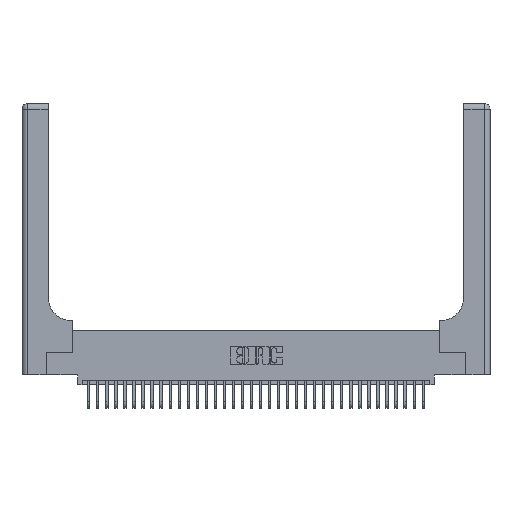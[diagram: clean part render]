
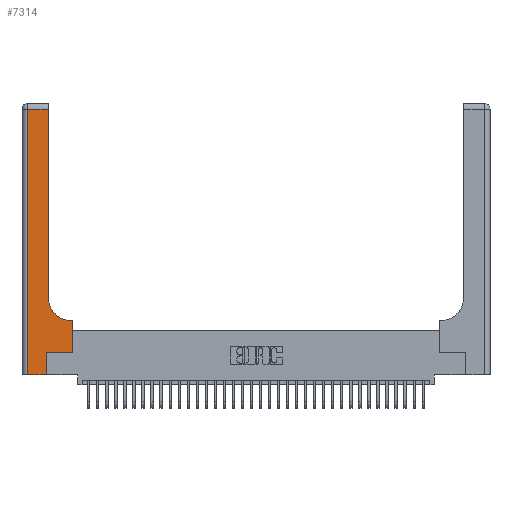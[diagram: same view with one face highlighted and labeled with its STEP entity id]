
A CAD part, top view. The second image highlights one B-rep face of the part: STEP entity #7314.
In plain terms, the highlighted planar face has unit normal (0, 0, 1).
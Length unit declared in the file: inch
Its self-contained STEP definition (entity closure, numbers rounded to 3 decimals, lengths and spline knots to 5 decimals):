
#1016 = ORIENTED_EDGE ( 'NONE', *, *, #7692, .T. ) ;
#1491 = CARTESIAN_POINT ( 'NONE',  ( 0.269, 0.25, 0.37 ) ) ;
#2041 = VERTEX_POINT ( 'NONE', #24677 ) ;
#3075 = EDGE_CURVE ( 'NONE', #2041, #9652, #34092, .T. ) ;
#4095 = DIRECTION ( 'NONE',  ( 1., 0., 0. ) ) ;
#4348 = LINE ( 'NONE', #24322, #18525 ) ;
#5325 = CARTESIAN_POINT ( 'NONE',  ( 0.5415, 0.85, 0.37 ) ) ;
#5831 = ORIENTED_EDGE ( 'NONE', *, *, #3075, .T. ) ;
#7272 = CARTESIAN_POINT ( 'NONE',  ( 0.5585, 0.25, 0.37 ) ) ;
#7314 = ADVANCED_FACE ( 'NONE', ( #29345 ), #9609, .F. ) ;
#7692 = EDGE_CURVE ( 'NONE', #11512, #23605, #4348, .T. ) ;
#8021 = DIRECTION ( 'NONE',  ( 1., 0., 0. ) ) ;
#8055 = ORIENTED_EDGE ( 'NONE', *, *, #15020, .T. ) ;
#8396 = DIRECTION ( 'NONE',  ( -1., 0., 0. ) ) ;
#9609 = PLANE ( 'NONE',  #15354 ) ;
#9652 = VERTEX_POINT ( 'NONE', #24457 ) ;
#10002 = VECTOR ( 'NONE', #10440, 39.37008 ) ;
#10163 = VECTOR ( 'NONE', #30963, 39.37008 ) ;
#10440 = DIRECTION ( 'NONE',  ( -1., 0., 0. ) ) ;
#11512 = VERTEX_POINT ( 'NONE', #14588 ) ;
#12380 = ORIENTED_EDGE ( 'NONE', *, *, #18925, .T. ) ;
#12418 = EDGE_CURVE ( 'NONE', #18332, #13739, #17398, .T. ) ;
#12611 = CARTESIAN_POINT ( 'NONE',  ( 0.269, 0., 0.37 ) ) ;
#12645 = DIRECTION ( 'NONE',  ( 0., 1., 0. ) ) ;
#13209 = CARTESIAN_POINT ( 'NONE',  ( 0., 2.94, 0.37 ) ) ;
#13588 = ORIENTED_EDGE ( 'NONE', *, *, #29686, .T. ) ;
#13739 = VERTEX_POINT ( 'NONE', #17241 ) ;
#14588 = CARTESIAN_POINT ( 'NONE',  ( 0.5585, 0.6, 0.37 ) ) ;
#14940 = CARTESIAN_POINT ( 'NONE',  ( 0., 3., 0.37 ) ) ;
#15020 = EDGE_CURVE ( 'NONE', #29560, #11512, #29086, .T. ) ;
#15139 = CARTESIAN_POINT ( 'NONE',  ( 0.06, 2.94, 0.37 ) ) ;
#15354 = AXIS2_PLACEMENT_3D ( 'NONE', #14940, #33501, #17611 ) ;
#15803 = DIRECTION ( 'NONE',  ( 0., 1., 0. ) ) ;
#16868 = CIRCLE ( 'NONE', #20278, 0.25 ) ;
#17241 = CARTESIAN_POINT ( 'NONE',  ( 0.269, 0.25, 0.37 ) ) ;
#17398 = LINE ( 'NONE', #26371, #30698 ) ;
#17611 = DIRECTION ( 'NONE',  ( -1., 0., 0. ) ) ;
#17655 = VECTOR ( 'NONE', #27578, 39.37008 ) ;
#17733 = CARTESIAN_POINT ( 'NONE',  ( 0.06, 3., 0.37 ) ) ;
#18332 = VERTEX_POINT ( 'NONE', #12611 ) ;
#18525 = VECTOR ( 'NONE', #8396, 39.37008 ) ;
#18925 = EDGE_CURVE ( 'NONE', #24624, #18332, #33434, .T. ) ;
#20275 = CARTESIAN_POINT ( 'NONE',  ( 0.2915, 3., 0.37 ) ) ;
#20278 = AXIS2_PLACEMENT_3D ( 'NONE', #5325, #23956, #8021 ) ;
#20395 = ORIENTED_EDGE ( 'NONE', *, *, #12418, .T. ) ;
#22029 = VECTOR ( 'NONE', #12645, 39.37008 ) ;
#23605 = VERTEX_POINT ( 'NONE', #27385 ) ;
#23956 = DIRECTION ( 'NONE',  ( 0., 0., -1. ) ) ;
#24119 = EDGE_CURVE ( 'NONE', #9652, #32865, #24959, .T. ) ;
#24322 = CARTESIAN_POINT ( 'NONE',  ( 0.2915, 0.6, 0.37 ) ) ;
#24457 = CARTESIAN_POINT ( 'NONE',  ( 0.2915, 2.94, 0.37 ) ) ;
#24624 = VERTEX_POINT ( 'NONE', #28833 ) ;
#24677 = CARTESIAN_POINT ( 'NONE',  ( 0.2915, 0.85, 0.37 ) ) ;
#24959 = LINE ( 'NONE', #13209, #10002 ) ;
#26371 = CARTESIAN_POINT ( 'NONE',  ( 0.269, 0., 0.37 ) ) ;
#26693 = EDGE_LOOP ( 'NONE', ( #5831, #28457, #27850, #12380, #20395, #13588, #8055, #1016, #27138 ) ) ;
#27138 = ORIENTED_EDGE ( 'NONE', *, *, #30465, .T. ) ;
#27385 = CARTESIAN_POINT ( 'NONE',  ( 0.5415, 0.6, 0.37 ) ) ;
#27474 = CARTESIAN_POINT ( 'NONE',  ( 0.5585, 0.25, 0.37 ) ) ;
#27578 = DIRECTION ( 'NONE',  ( 1., 0., 0. ) ) ;
#27850 = ORIENTED_EDGE ( 'NONE', *, *, #31530, .T. ) ;
#28457 = ORIENTED_EDGE ( 'NONE', *, *, #24119, .T. ) ;
#28558 = VECTOR ( 'NONE', #4095, 39.37008 ) ;
#28833 = CARTESIAN_POINT ( 'NONE',  ( 0.06, 0., 0.37 ) ) ;
#29086 = LINE ( 'NONE', #7272, #22029 ) ;
#29345 = FACE_OUTER_BOUND ( 'NONE', #26693, .T. ) ;
#29394 = LINE ( 'NONE', #1491, #28558 ) ;
#29560 = VERTEX_POINT ( 'NONE', #27474 ) ;
#29686 = EDGE_CURVE ( 'NONE', #13739, #29560, #29394, .T. ) ;
#30465 = EDGE_CURVE ( 'NONE', #23605, #2041, #16868, .T. ) ;
#30488 = LINE ( 'NONE', #17733, #10163 ) ;
#30698 = VECTOR ( 'NONE', #15803, 39.37008 ) ;
#30963 = DIRECTION ( 'NONE',  ( 0., -1., 0. ) ) ;
#31530 = EDGE_CURVE ( 'NONE', #32865, #24624, #30488, .T. ) ;
#32865 = VERTEX_POINT ( 'NONE', #15139 ) ;
#32911 = CARTESIAN_POINT ( 'NONE',  ( 0., 0., 0.37 ) ) ;
#33266 = VECTOR ( 'NONE', #33508, 39.37008 ) ;
#33434 = LINE ( 'NONE', #32911, #17655 ) ;
#33501 = DIRECTION ( 'NONE',  ( 0., 0., -1. ) ) ;
#33508 = DIRECTION ( 'NONE',  ( 0., 1., 0. ) ) ;
#34092 = LINE ( 'NONE', #20275, #33266 ) ;
